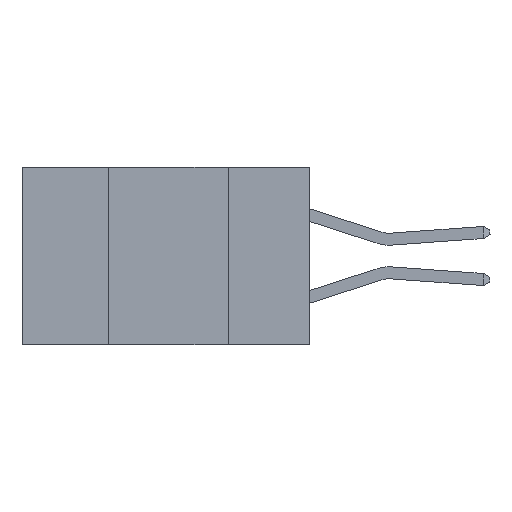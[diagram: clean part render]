
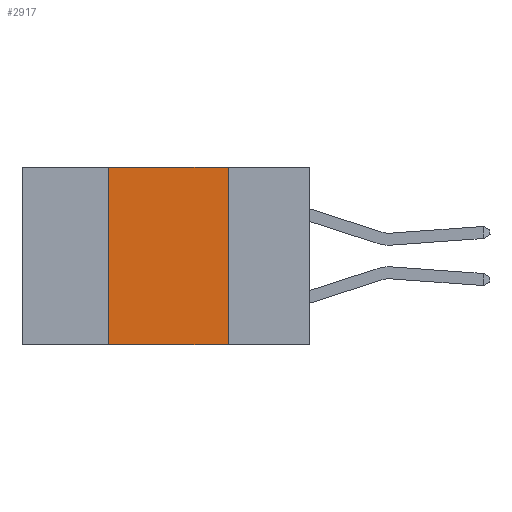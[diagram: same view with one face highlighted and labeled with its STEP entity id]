
A CAD part, left-side view. The second image highlights one B-rep face of the part: STEP entity #2917.
In plain terms, the highlighted planar face has unit normal (-1, 0, 0).
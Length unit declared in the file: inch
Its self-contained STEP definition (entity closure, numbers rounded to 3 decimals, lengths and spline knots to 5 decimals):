
#75 = CARTESIAN_POINT ( 'NONE',  ( 0., 0.6, 0. ) ) ;
#563 = CARTESIAN_POINT ( 'NONE',  ( 0., 0.42, 0. ) ) ;
#688 = LINE ( 'NONE', #2278, #10271 ) ;
#740 = LINE ( 'NONE', #75, #2306 ) ;
#792 = EDGE_LOOP ( 'NONE', ( #9396, #6659, #1959, #5987 ) ) ;
#972 = EDGE_CURVE ( 'NONE', #9621, #2172, #6798, .T. ) ;
#1183 = VERTEX_POINT ( 'NONE', #4762 ) ;
#1729 = CARTESIAN_POINT ( 'NONE',  ( 0., 0.6, 0. ) ) ;
#1959 = ORIENTED_EDGE ( 'NONE', *, *, #2774, .F. ) ;
#2172 = VERTEX_POINT ( 'NONE', #9194 ) ;
#2177 = EDGE_CURVE ( 'NONE', #1183, #2172, #9945, .T. ) ;
#2278 = CARTESIAN_POINT ( 'NONE',  ( 0., 0.42, -0.37 ) ) ;
#2306 = VECTOR ( 'NONE', #9912, 39.37008 ) ;
#2774 = EDGE_CURVE ( 'NONE', #9621, #6861, #688, .T. ) ;
#2917 = ADVANCED_FACE ( 'NONE', ( #8412 ), #5074, .F. ) ;
#3335 = CARTESIAN_POINT ( 'NONE',  ( 0., 0.17, -0.37 ) ) ;
#3559 = CARTESIAN_POINT ( 'NONE',  ( 0., 0.6, -0.37 ) ) ;
#3796 = VECTOR ( 'NONE', #9344, 39.37008 ) ;
#4762 = CARTESIAN_POINT ( 'NONE',  ( 0., 0.17, 0. ) ) ;
#4806 = VECTOR ( 'NONE', #10211, 39.37008 ) ;
#5074 = PLANE ( 'NONE',  #7867 ) ;
#5987 = ORIENTED_EDGE ( 'NONE', *, *, #972, .T. ) ;
#6659 = ORIENTED_EDGE ( 'NONE', *, *, #9075, .F. ) ;
#6798 = LINE ( 'NONE', #3559, #4806 ) ;
#6861 = VERTEX_POINT ( 'NONE', #563 ) ;
#7867 = AXIS2_PLACEMENT_3D ( 'NONE', #1729, #10076, #8518 ) ;
#8412 = FACE_OUTER_BOUND ( 'NONE', #792, .T. ) ;
#8518 = DIRECTION ( 'NONE',  ( 0., 0., -1. ) ) ;
#8746 = CARTESIAN_POINT ( 'NONE',  ( 0., 0.42, -0.37 ) ) ;
#9010 = DIRECTION ( 'NONE',  ( 0., 0., 1. ) ) ;
#9075 = EDGE_CURVE ( 'NONE', #6861, #1183, #740, .T. ) ;
#9194 = CARTESIAN_POINT ( 'NONE',  ( 0., 0.17, -0.37 ) ) ;
#9344 = DIRECTION ( 'NONE',  ( 0., 0., -1. ) ) ;
#9396 = ORIENTED_EDGE ( 'NONE', *, *, #2177, .F. ) ;
#9621 = VERTEX_POINT ( 'NONE', #8746 ) ;
#9912 = DIRECTION ( 'NONE',  ( 0., -1., 0. ) ) ;
#9945 = LINE ( 'NONE', #3335, #3796 ) ;
#10076 = DIRECTION ( 'NONE',  ( 1., 0., 0. ) ) ;
#10211 = DIRECTION ( 'NONE',  ( 0., -1., 0. ) ) ;
#10271 = VECTOR ( 'NONE', #9010, 39.37008 ) ;
